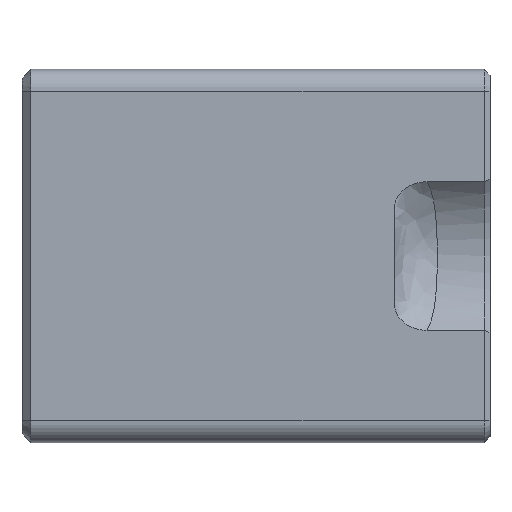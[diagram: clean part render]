
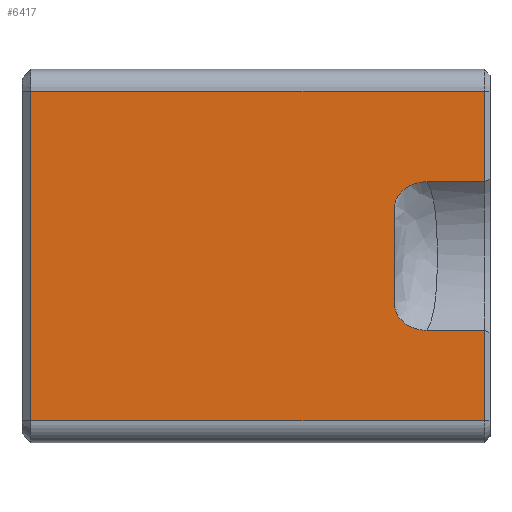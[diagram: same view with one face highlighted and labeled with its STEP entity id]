
A CAD part, front view. The second image highlights one B-rep face of the part: STEP entity #6417.
In plain terms, the highlighted planar face has unit normal (0, -1, 0).
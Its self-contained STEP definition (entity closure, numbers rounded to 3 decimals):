
#551=B_SPLINE_CURVE_WITH_KNOTS('',3,(#15637,#15638,#15639,#15640,#15641,
#15642,#15643,#15644,#15645,#15646,#15647,#15648,#15649,#15650,#15651,#15652,
#15653,#15654,#15655,#15656),.UNSPECIFIED.,.F.,.F.,(4,2,2,2,2,2,2,2,2,4),
(0.,0.,0.,0.002,0.007,
0.018,0.04,0.085,0.157,
0.234),.UNSPECIFIED.);
#552=B_SPLINE_CURVE_WITH_KNOTS('',3,(#15660,#15661,#15662,#15663,#15664,
#15665,#15666,#15667,#15668,#15669,#15670,#15671,#15672,#15673,#15674,#15675,
#15676,#15677,#15678,#15679),.UNSPECIFIED.,.F.,.F.,(4,2,2,2,2,2,2,2,2,4),
(0.,0.102,0.197,0.257,0.286,
0.3,0.306,0.31,0.31,
0.31),.UNSPECIFIED.);
#717=PLANE('',#6913);
#1161=FACE_OUTER_BOUND('',#1556,.T.);
#1556=EDGE_LOOP('',(#5959,#5960,#5961,#5962,#5963,#5964,#5965,#5966,#5967,
#5968));
#1904=LINE('',#15604,#2261);
#1913=LINE('',#15626,#2270);
#1914=LINE('',#15631,#2271);
#1915=LINE('',#15635,#2272);
#1916=LINE('',#15658,#2273);
#1917=LINE('',#15680,#2274);
#1918=LINE('',#15682,#2275);
#1919=LINE('',#15683,#2276);
#2261=VECTOR('',#8140,10.);
#2270=VECTOR('',#8173,10.);
#2271=VECTOR('',#8180,10.);
#2272=VECTOR('',#8185,10.);
#2273=VECTOR('',#8186,10.);
#2274=VECTOR('',#8187,10.);
#2275=VECTOR('',#8188,10.);
#2276=VECTOR('',#8189,10.);
#3100=VERTEX_POINT('',#15591);
#3101=VERTEX_POINT('',#15596);
#3102=VERTEX_POINT('',#15603);
#3103=VERTEX_POINT('',#15622);
#3104=VERTEX_POINT('',#15630);
#3105=VERTEX_POINT('',#15634);
#3106=VERTEX_POINT('',#15636);
#3107=VERTEX_POINT('',#15657);
#3108=VERTEX_POINT('',#15659);
#3109=VERTEX_POINT('',#15681);
#4048=EDGE_CURVE('',#3101,#3102,#1904,.T.);
#4061=EDGE_CURVE('',#3103,#3100,#1913,.T.);
#4063=EDGE_CURVE('',#3102,#3104,#1914,.T.);
#4065=EDGE_CURVE('',#3101,#3105,#1915,.T.);
#4066=EDGE_CURVE('',#3106,#3105,#551,.T.);
#4067=EDGE_CURVE('',#3106,#3107,#1916,.T.);
#4068=EDGE_CURVE('',#3107,#3108,#552,.F.);
#4069=EDGE_CURVE('',#3108,#3100,#1917,.T.);
#4070=EDGE_CURVE('',#3109,#3103,#1918,.T.);
#4071=EDGE_CURVE('',#3104,#3109,#1919,.T.);
#5959=ORIENTED_EDGE('',*,*,#4048,.F.);
#5960=ORIENTED_EDGE('',*,*,#4065,.T.);
#5961=ORIENTED_EDGE('',*,*,#4066,.F.);
#5962=ORIENTED_EDGE('',*,*,#4067,.T.);
#5963=ORIENTED_EDGE('',*,*,#4068,.T.);
#5964=ORIENTED_EDGE('',*,*,#4069,.T.);
#5965=ORIENTED_EDGE('',*,*,#4061,.F.);
#5966=ORIENTED_EDGE('',*,*,#4070,.F.);
#5967=ORIENTED_EDGE('',*,*,#4071,.F.);
#5968=ORIENTED_EDGE('',*,*,#4063,.F.);
#6417=ADVANCED_FACE('',(#1161),#717,.T.);
#6913=AXIS2_PLACEMENT_3D('',#15633,#8183,#8184);
#8140=DIRECTION('',(0.,0.,-1.));
#8173=DIRECTION('',(0.,0.,-1.));
#8180=DIRECTION('',(-1.,0.,0.));
#8183=DIRECTION('center_axis',(0.,-1.,0.));
#8184=DIRECTION('ref_axis',(0.,0.,1.));
#8185=DIRECTION('',(-1.,0.,0.));
#8186=DIRECTION('',(0.,0.,1.));
#8187=DIRECTION('',(1.,0.,0.));
#8188=DIRECTION('',(1.,0.,0.));
#8189=DIRECTION('',(0.,0.,1.));
#15591=CARTESIAN_POINT('',(-183.534,-11.455,5.083));
#15596=CARTESIAN_POINT('',(-183.534,-11.455,-5.083));
#15603=CARTESIAN_POINT('',(-183.534,-11.455,-11.264));
#15604=CARTESIAN_POINT('',(-183.534,-11.455,-6.128));
#15622=CARTESIAN_POINT('',(-183.534,-11.455,11.264));
#15626=CARTESIAN_POINT('',(-183.534,-11.455,-6.128));
#15630=CARTESIAN_POINT('',(-214.534,-11.455,-11.264));
#15631=CARTESIAN_POINT('',(-183.134,-11.455,-11.264));
#15633=CARTESIAN_POINT('Origin',(-183.134,-11.455,-12.256));
#15634=CARTESIAN_POINT('',(-187.44,-11.455,-5.083));
#15635=CARTESIAN_POINT('',(-183.134,-11.455,-5.083));
#15636=CARTESIAN_POINT('',(-189.634,-11.455,-3.546));
#15637=CARTESIAN_POINT('Ctrl Pts',(-189.634,-11.455,-3.546));
#15638=CARTESIAN_POINT('Ctrl Pts',(-189.634,-11.455,-3.546));
#15639=CARTESIAN_POINT('Ctrl Pts',(-189.634,-11.455,-3.547));
#15640=CARTESIAN_POINT('Ctrl Pts',(-189.634,-11.455,-3.548));
#15641=CARTESIAN_POINT('Ctrl Pts',(-189.634,-11.455,-3.549));
#15642=CARTESIAN_POINT('Ctrl Pts',(-189.634,-11.455,-3.558));
#15643=CARTESIAN_POINT('Ctrl Pts',(-189.633,-11.455,-3.566));
#15644=CARTESIAN_POINT('Ctrl Pts',(-189.63,-11.455,-3.592));
#15645=CARTESIAN_POINT('Ctrl Pts',(-189.627,-11.455,-3.61));
#15646=CARTESIAN_POINT('Ctrl Pts',(-189.616,-11.455,-3.667));
#15647=CARTESIAN_POINT('Ctrl Pts',(-189.605,-11.455,-3.707));
#15648=CARTESIAN_POINT('Ctrl Pts',(-189.566,-11.455,-3.826));
#15649=CARTESIAN_POINT('Ctrl Pts',(-189.531,-11.455,-3.905));
#15650=CARTESIAN_POINT('Ctrl Pts',(-189.407,-11.455,-4.136));
#15651=CARTESIAN_POINT('Ctrl Pts',(-189.297,-11.455,
-4.279));
#15652=CARTESIAN_POINT('Ctrl Pts',(-188.973,-11.455,
-4.603));
#15653=CARTESIAN_POINT('Ctrl Pts',(-188.724,-11.455,-4.771));
#15654=CARTESIAN_POINT('Ctrl Pts',(-188.119,-11.455,-5.02));
#15655=CARTESIAN_POINT('Ctrl Pts',(-187.781,-11.455,-5.083));
#15656=CARTESIAN_POINT('Ctrl Pts',(-187.44,-11.455,-5.083));
#15657=CARTESIAN_POINT('',(-189.634,-11.455,3.546));
#15658=CARTESIAN_POINT('',(-189.634,-11.455,-6.128));
#15659=CARTESIAN_POINT('',(-187.44,-11.455,5.083));
#15660=CARTESIAN_POINT('Ctrl Pts',(-187.44,-11.455,5.083));
#15661=CARTESIAN_POINT('Ctrl Pts',(-187.781,-11.455,5.083));
#15662=CARTESIAN_POINT('Ctrl Pts',(-188.119,-11.455,5.02));
#15663=CARTESIAN_POINT('Ctrl Pts',(-188.724,-11.455,4.771));
#15664=CARTESIAN_POINT('Ctrl Pts',(-188.973,-11.455,
4.603));
#15665=CARTESIAN_POINT('Ctrl Pts',(-189.297,-11.455,
4.279));
#15666=CARTESIAN_POINT('Ctrl Pts',(-189.407,-11.455,4.136));
#15667=CARTESIAN_POINT('Ctrl Pts',(-189.531,-11.455,3.905));
#15668=CARTESIAN_POINT('Ctrl Pts',(-189.566,-11.455,3.826));
#15669=CARTESIAN_POINT('Ctrl Pts',(-189.605,-11.455,3.707));
#15670=CARTESIAN_POINT('Ctrl Pts',(-189.616,-11.455,3.667));
#15671=CARTESIAN_POINT('Ctrl Pts',(-189.627,-11.455,3.61));
#15672=CARTESIAN_POINT('Ctrl Pts',(-189.63,-11.455,3.592));
#15673=CARTESIAN_POINT('Ctrl Pts',(-189.633,-11.455,3.565));
#15674=CARTESIAN_POINT('Ctrl Pts',(-189.634,-11.455,3.557));
#15675=CARTESIAN_POINT('Ctrl Pts',(-189.634,-11.455,3.549));
#15676=CARTESIAN_POINT('Ctrl Pts',(-189.634,-11.455,3.548));
#15677=CARTESIAN_POINT('Ctrl Pts',(-189.634,-11.455,3.547));
#15678=CARTESIAN_POINT('Ctrl Pts',(-189.634,-11.455,3.546));
#15679=CARTESIAN_POINT('Ctrl Pts',(-189.634,-11.455,3.546));
#15680=CARTESIAN_POINT('',(-183.134,-11.455,5.083));
#15681=CARTESIAN_POINT('',(-214.534,-11.455,11.264));
#15682=CARTESIAN_POINT('',(-183.134,-11.455,11.264));
#15683=CARTESIAN_POINT('',(-214.534,-11.455,-6.128));
